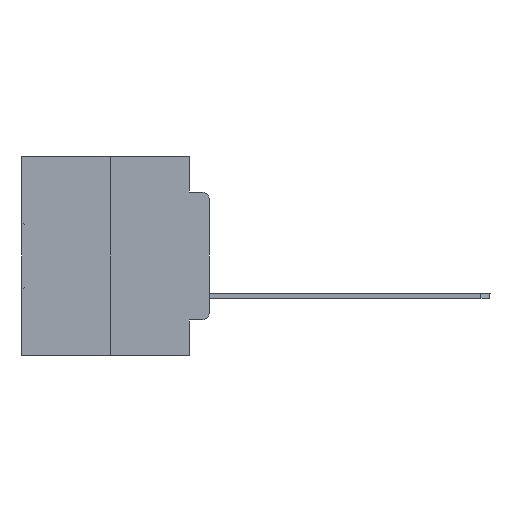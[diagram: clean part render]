
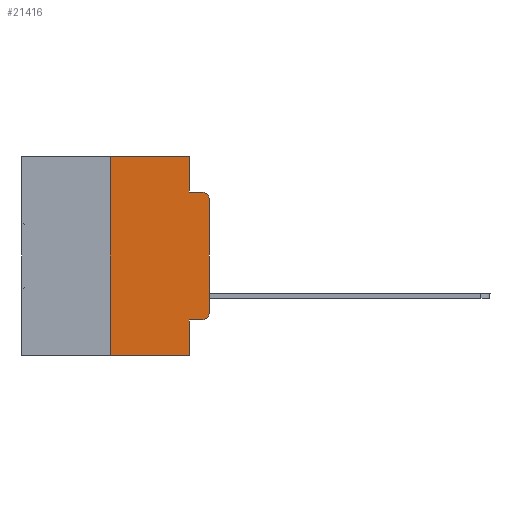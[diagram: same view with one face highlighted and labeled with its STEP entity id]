
A CAD part, left-side view. The second image highlights one B-rep face of the part: STEP entity #21416.
In plain terms, the highlighted planar face has unit normal (-1, 0, 0).
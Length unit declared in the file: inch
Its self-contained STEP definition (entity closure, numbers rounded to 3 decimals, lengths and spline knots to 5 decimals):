
#56 = DIRECTION ( 'NONE',  ( 0., -1., 0. ) ) ;
#451 = DIRECTION ( 'NONE',  ( 1., 0., 0. ) ) ;
#459 = VECTOR ( 'NONE', #10718, 39.37008 ) ;
#1206 = CARTESIAN_POINT ( 'NONE',  ( 0., 0.051, 0. ) ) ;
#1276 = VECTOR ( 'NONE', #17138, 39.37008 ) ;
#1846 = CARTESIAN_POINT ( 'NONE',  ( 0., 0.02, -0.0885 ) ) ;
#1914 = AXIS2_PLACEMENT_3D ( 'NONE', #15696, #22411, #15222 ) ;
#2062 = EDGE_CURVE ( 'NONE', #25764, #10123, #16361, .T. ) ;
#2368 = EDGE_CURVE ( 'NONE', #22502, #21797, #13121, .T. ) ;
#2668 = CARTESIAN_POINT ( 'NONE',  ( 0., 0.25, -0.5 ) ) ;
#2950 = ORIENTED_EDGE ( 'NONE', *, *, #3963, .T. ) ;
#3714 = ORIENTED_EDGE ( 'NONE', *, *, #2368, .T. ) ;
#3757 = EDGE_LOOP ( 'NONE', ( #2950, #24308, #8431, #4905, #31186, #30962, #19637, #6940, #8224, #3714 ) ) ;
#3761 = CARTESIAN_POINT ( 'NONE',  ( 0., 0.473, -0.5 ) ) ;
#3963 = EDGE_CURVE ( 'NONE', #21797, #31477, #30200, .T. ) ;
#4081 = DIRECTION ( 'NONE',  ( 0., -1., 0. ) ) ;
#4905 = ORIENTED_EDGE ( 'NONE', *, *, #12943, .F. ) ;
#6073 = LINE ( 'NONE', #27044, #459 ) ;
#6142 = DIRECTION ( 'NONE',  ( -1., 0., 0. ) ) ;
#6206 = DIRECTION ( 'NONE',  ( 0., 0., -1. ) ) ;
#6734 = EDGE_CURVE ( 'NONE', #31477, #7900, #16924, .T. ) ;
#6940 = ORIENTED_EDGE ( 'NONE', *, *, #8976, .F. ) ;
#7051 = VERTEX_POINT ( 'NONE', #8189 ) ;
#7232 = CARTESIAN_POINT ( 'NONE',  ( 0., 0.051, -0.4115 ) ) ;
#7861 = CARTESIAN_POINT ( 'NONE',  ( 0., 0., -0.1085 ) ) ;
#7900 = VERTEX_POINT ( 'NONE', #1846 ) ;
#8189 = CARTESIAN_POINT ( 'NONE',  ( 0., 0.25, 0. ) ) ;
#8224 = ORIENTED_EDGE ( 'NONE', *, *, #30315, .T. ) ;
#8431 = ORIENTED_EDGE ( 'NONE', *, *, #16326, .F. ) ;
#8976 = EDGE_CURVE ( 'NONE', #29542, #10123, #21213, .T. ) ;
#9178 = DIRECTION ( 'NONE',  ( 0., 0., -1. ) ) ;
#9493 = LINE ( 'NONE', #24160, #1276 ) ;
#10123 = VERTEX_POINT ( 'NONE', #27646 ) ;
#10186 = DIRECTION ( 'NONE',  ( 0., 0., -1. ) ) ;
#10718 = DIRECTION ( 'NONE',  ( 0., -1., 0. ) ) ;
#11173 = EDGE_CURVE ( 'NONE', #7051, #30674, #18897, .T. ) ;
#11303 = EDGE_CURVE ( 'NONE', #25764, #7051, #9493, .T. ) ;
#11482 = VECTOR ( 'NONE', #20822, 39.37008 ) ;
#12500 = VECTOR ( 'NONE', #25614, 39.37008 ) ;
#12578 = CARTESIAN_POINT ( 'NONE',  ( 0., 0.473, 0. ) ) ;
#12943 = EDGE_CURVE ( 'NONE', #30674, #27028, #25456, .T. ) ;
#13121 = CIRCLE ( 'NONE', #1914, 0.02 ) ;
#13197 = CARTESIAN_POINT ( 'NONE',  ( 0., 0.051, -0.4115 ) ) ;
#13214 = VECTOR ( 'NONE', #29895, 39.37008 ) ;
#15042 = VECTOR ( 'NONE', #56, 39.37008 ) ;
#15222 = DIRECTION ( 'NONE',  ( 0., 0., -1. ) ) ;
#15696 = CARTESIAN_POINT ( 'NONE',  ( 0., 0.02, -0.3915 ) ) ;
#16326 = EDGE_CURVE ( 'NONE', #27028, #7900, #6073, .T. ) ;
#16361 = LINE ( 'NONE', #3761, #24770 ) ;
#16924 = CIRCLE ( 'NONE', #28141, 0.02 ) ;
#17138 = DIRECTION ( 'NONE',  ( 0., 0., 1. ) ) ;
#17982 = PLANE ( 'NONE',  #23139 ) ;
#18897 = LINE ( 'NONE', #28638, #11482 ) ;
#19295 = CARTESIAN_POINT ( 'NONE',  ( 0., 0.02, -0.4115 ) ) ;
#19637 = ORIENTED_EDGE ( 'NONE', *, *, #2062, .T. ) ;
#19722 = CARTESIAN_POINT ( 'NONE',  ( 0., 0., -0.3915 ) ) ;
#20458 = CARTESIAN_POINT ( 'NONE',  ( 0., 0., 0. ) ) ;
#20822 = DIRECTION ( 'NONE',  ( 0., -1., 0. ) ) ;
#21213 = LINE ( 'NONE', #26150, #27674 ) ;
#21416 = ADVANCED_FACE ( 'NONE', ( #22785 ), #17982, .F. ) ;
#21797 = VERTEX_POINT ( 'NONE', #19722 ) ;
#22411 = DIRECTION ( 'NONE',  ( -1., 0., 0. ) ) ;
#22477 = CARTESIAN_POINT ( 'NONE',  ( 0., 0.051, 0. ) ) ;
#22502 = VERTEX_POINT ( 'NONE', #19295 ) ;
#22666 = LINE ( 'NONE', #7232, #15042 ) ;
#22785 = FACE_OUTER_BOUND ( 'NONE', #3757, .T. ) ;
#23139 = AXIS2_PLACEMENT_3D ( 'NONE', #12578, #451, #10186 ) ;
#24160 = CARTESIAN_POINT ( 'NONE',  ( 0., 0.25, 0. ) ) ;
#24308 = ORIENTED_EDGE ( 'NONE', *, *, #6734, .T. ) ;
#24770 = VECTOR ( 'NONE', #4081, 39.37008 ) ;
#25456 = LINE ( 'NONE', #1206, #12500 ) ;
#25614 = DIRECTION ( 'NONE',  ( 0., 0., -1. ) ) ;
#25764 = VERTEX_POINT ( 'NONE', #2668 ) ;
#26150 = CARTESIAN_POINT ( 'NONE',  ( 0., 0.051, 0. ) ) ;
#27028 = VERTEX_POINT ( 'NONE', #27255 ) ;
#27044 = CARTESIAN_POINT ( 'NONE',  ( 0., 0.051, -0.0885 ) ) ;
#27255 = CARTESIAN_POINT ( 'NONE',  ( 0., 0.051, -0.0885 ) ) ;
#27646 = CARTESIAN_POINT ( 'NONE',  ( 0., 0.051, -0.5 ) ) ;
#27674 = VECTOR ( 'NONE', #6206, 39.37008 ) ;
#28141 = AXIS2_PLACEMENT_3D ( 'NONE', #28341, #6142, #9178 ) ;
#28341 = CARTESIAN_POINT ( 'NONE',  ( 0., 0.02, -0.1085 ) ) ;
#28638 = CARTESIAN_POINT ( 'NONE',  ( 0., 0.473, 0. ) ) ;
#29542 = VERTEX_POINT ( 'NONE', #13197 ) ;
#29895 = DIRECTION ( 'NONE',  ( 0., 0., 1. ) ) ;
#30200 = LINE ( 'NONE', #20458, #13214 ) ;
#30315 = EDGE_CURVE ( 'NONE', #29542, #22502, #22666, .T. ) ;
#30674 = VERTEX_POINT ( 'NONE', #22477 ) ;
#30962 = ORIENTED_EDGE ( 'NONE', *, *, #11303, .F. ) ;
#31186 = ORIENTED_EDGE ( 'NONE', *, *, #11173, .F. ) ;
#31477 = VERTEX_POINT ( 'NONE', #7861 ) ;
